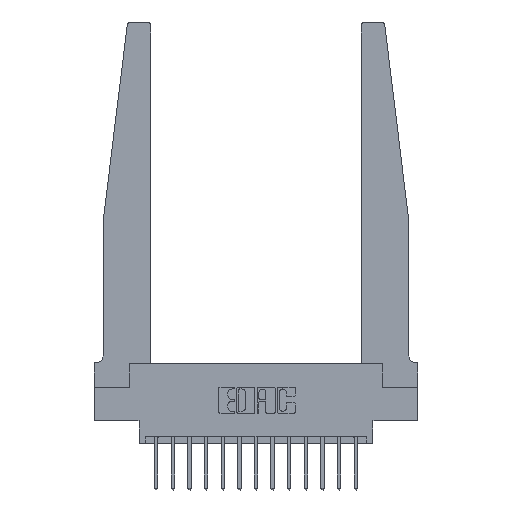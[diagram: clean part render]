
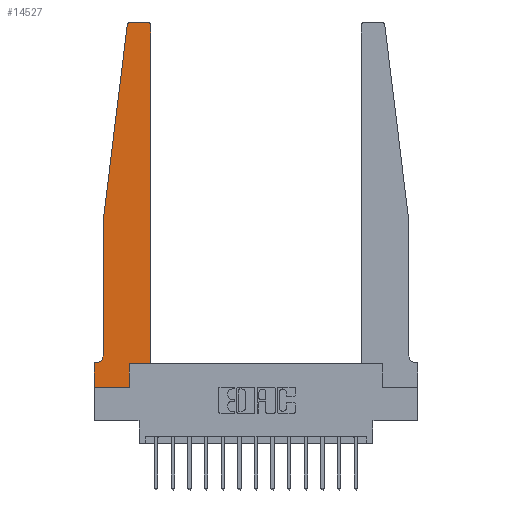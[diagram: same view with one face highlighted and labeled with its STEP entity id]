
A CAD part, top view. The second image highlights one B-rep face of the part: STEP entity #14527.
In plain terms, the highlighted planar face has unit normal (0, 0, 1).
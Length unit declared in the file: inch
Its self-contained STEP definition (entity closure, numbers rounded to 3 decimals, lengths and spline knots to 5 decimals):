
#249 = CARTESIAN_POINT ( 'NONE',  ( 0.2605, 0.18, 0.37 ) ) ;
#412 = VERTEX_POINT ( 'NONE', #7031 ) ;
#524 = DIRECTION ( 'NONE',  ( 1., 0., 0. ) ) ;
#553 = DIRECTION ( 'NONE',  ( -1., 0., 0. ) ) ;
#1362 = LINE ( 'NONE', #14492, #8134 ) ;
#2396 = CARTESIAN_POINT ( 'NONE',  ( 0.27653, 2.72, 0.37 ) ) ;
#2543 = DIRECTION ( 'NONE',  ( 1., 0., 0. ) ) ;
#2565 = VERTEX_POINT ( 'NONE', #249 ) ;
#2667 = EDGE_LOOP ( 'NONE', ( #16697, #17118, #3313, #10289, #3746, #11726, #4587, #15680, #12146, #9450, #15894, #10908 ) ) ;
#2703 = DIRECTION ( 'NONE',  ( 0., 0., -1. ) ) ;
#2817 = VECTOR ( 'NONE', #12743, 39.37008 ) ;
#2954 = AXIS2_PLACEMENT_3D ( 'NONE', #10752, #2703, #12099 ) ;
#3021 = EDGE_CURVE ( 'NONE', #12821, #3714, #10484, .T. ) ;
#3313 = ORIENTED_EDGE ( 'NONE', *, *, #9236, .T. ) ;
#3453 = VECTOR ( 'NONE', #9920, 39.37008 ) ;
#3548 = LINE ( 'NONE', #11405, #10287 ) ;
#3714 = VERTEX_POINT ( 'NONE', #16262 ) ;
#3727 = FACE_OUTER_BOUND ( 'NONE', #2667, .T. ) ;
#3746 = ORIENTED_EDGE ( 'NONE', *, *, #3021, .T. ) ;
#3760 = DIRECTION ( 'NONE',  ( 1., 0., 0. ) ) ;
#4009 = DIRECTION ( 'NONE',  ( 0., -1., 0. ) ) ;
#4229 = VERTEX_POINT ( 'NONE', #16012 ) ;
#4432 = VERTEX_POINT ( 'NONE', #14470 ) ;
#4587 = ORIENTED_EDGE ( 'NONE', *, *, #8149, .T. ) ;
#4724 = CARTESIAN_POINT ( 'NONE',  ( 0.2605, 0.18, 0.37 ) ) ;
#4730 = LINE ( 'NONE', #10599, #11858 ) ;
#5122 = EDGE_CURVE ( 'NONE', #2565, #16673, #4730, .T. ) ;
#5368 = VERTEX_POINT ( 'NONE', #8554 ) ;
#5575 = EDGE_CURVE ( 'NONE', #4432, #5368, #1362, .T. ) ;
#5915 = LINE ( 'NONE', #12047, #12614 ) ;
#6221 = VERTEX_POINT ( 'NONE', #14526 ) ;
#6348 = VECTOR ( 'NONE', #15197, 39.37008 ) ;
#6375 = CIRCLE ( 'NONE', #12359, 0.03 ) ;
#6402 = VERTEX_POINT ( 'NONE', #6806 ) ;
#6451 = EDGE_CURVE ( 'NONE', #16673, #6221, #14570, .T. ) ;
#6667 = AXIS2_PLACEMENT_3D ( 'NONE', #7241, #8604, #524 ) ;
#6700 = DIRECTION ( 'NONE',  ( 0., 0., 1. ) ) ;
#6715 = EDGE_CURVE ( 'NONE', #5368, #2565, #6821, .T. ) ;
#6806 = CARTESIAN_POINT ( 'NONE',  ( 0., 0.1875, 0.37 ) ) ;
#6821 = LINE ( 'NONE', #4724, #2817 ) ;
#6932 = AXIS2_PLACEMENT_3D ( 'NONE', #2396, #11792, #3760 ) ;
#7011 = CARTESIAN_POINT ( 'NONE',  ( 0.065, 0.2375, 0.37 ) ) ;
#7031 = CARTESIAN_POINT ( 'NONE',  ( 0.24675, 2.72367, 0.37 ) ) ;
#7032 = LINE ( 'NONE', #15213, #3453 ) ;
#7241 = CARTESIAN_POINT ( 'NONE',  ( 0., 0.1875, 0.37 ) ) ;
#7588 = EDGE_CURVE ( 'NONE', #12906, #11957, #15149, .T. ) ;
#7838 = DIRECTION ( 'NONE',  ( 1., 0., 0. ) ) ;
#8134 = VECTOR ( 'NONE', #7838, 39.37008 ) ;
#8149 = EDGE_CURVE ( 'NONE', #6402, #4432, #10353, .T. ) ;
#8226 = CARTESIAN_POINT ( 'NONE',  ( 0.425, 0.18, 0.37 ) ) ;
#8378 = CIRCLE ( 'NONE', #6932, 0.03 ) ;
#8470 = CARTESIAN_POINT ( 'NONE',  ( 0.27653, 2.75, 0.37 ) ) ;
#8554 = CARTESIAN_POINT ( 'NONE',  ( 0.2605, 0., 0.37 ) ) ;
#8604 = DIRECTION ( 'NONE',  ( 0., 0., 1. ) ) ;
#9236 = EDGE_CURVE ( 'NONE', #412, #4229, #7032, .T. ) ;
#9450 = ORIENTED_EDGE ( 'NONE', *, *, #5122, .T. ) ;
#9846 = CARTESIAN_POINT ( 'NONE',  ( 0., 0., 0.37 ) ) ;
#9920 = DIRECTION ( 'NONE',  ( -0.122, -0.992, 0. ) ) ;
#10068 = EDGE_CURVE ( 'NONE', #6221, #12906, #6375, .T. ) ;
#10287 = VECTOR ( 'NONE', #12667, 39.37008 ) ;
#10289 = ORIENTED_EDGE ( 'NONE', *, *, #11103, .T. ) ;
#10353 = LINE ( 'NONE', #9846, #6348 ) ;
#10484 = CIRCLE ( 'NONE', #2954, 0.05 ) ;
#10599 = CARTESIAN_POINT ( 'NONE',  ( 0.425, 0.18, 0.37 ) ) ;
#10752 = CARTESIAN_POINT ( 'NONE',  ( 0.015, 0.2375, 0.37 ) ) ;
#10902 = DIRECTION ( 'NONE',  ( 0., 1., 0. ) ) ;
#10908 = ORIENTED_EDGE ( 'NONE', *, *, #10068, .T. ) ;
#11103 = EDGE_CURVE ( 'NONE', #4229, #12821, #5915, .T. ) ;
#11405 = CARTESIAN_POINT ( 'NONE',  ( 0.065, 0.1875, 0.37 ) ) ;
#11726 = ORIENTED_EDGE ( 'NONE', *, *, #12977, .T. ) ;
#11792 = DIRECTION ( 'NONE',  ( 0., 0., 1. ) ) ;
#11804 = CARTESIAN_POINT ( 'NONE',  ( 0.425, 0.18, 0.37 ) ) ;
#11858 = VECTOR ( 'NONE', #2543, 39.37008 ) ;
#11957 = VERTEX_POINT ( 'NONE', #8470 ) ;
#12047 = CARTESIAN_POINT ( 'NONE',  ( 0.065, 1.25, 0.37 ) ) ;
#12099 = DIRECTION ( 'NONE',  ( -1., 0., 0. ) ) ;
#12146 = ORIENTED_EDGE ( 'NONE', *, *, #6715, .T. ) ;
#12359 = AXIS2_PLACEMENT_3D ( 'NONE', #14709, #6700, #16029 ) ;
#12614 = VECTOR ( 'NONE', #4009, 39.37008 ) ;
#12667 = DIRECTION ( 'NONE',  ( -1., 0., 0. ) ) ;
#12743 = DIRECTION ( 'NONE',  ( 0., 1., 0. ) ) ;
#12821 = VERTEX_POINT ( 'NONE', #7011 ) ;
#12906 = VERTEX_POINT ( 'NONE', #16514 ) ;
#12977 = EDGE_CURVE ( 'NONE', #3714, #6402, #3548, .T. ) ;
#13300 = VECTOR ( 'NONE', #10902, 39.37008 ) ;
#14331 = VECTOR ( 'NONE', #553, 39.37008 ) ;
#14470 = CARTESIAN_POINT ( 'NONE',  ( 0., 0., 0.37 ) ) ;
#14492 = CARTESIAN_POINT ( 'NONE',  ( 0., 0., 0.37 ) ) ;
#14526 = CARTESIAN_POINT ( 'NONE',  ( 0.425, 2.72, 0.37 ) ) ;
#14527 = ADVANCED_FACE ( 'NONE', ( #3727 ), #15239, .T. ) ;
#14570 = LINE ( 'NONE', #8226, #13300 ) ;
#14709 = CARTESIAN_POINT ( 'NONE',  ( 0.395, 2.72, 0.37 ) ) ;
#15149 = LINE ( 'NONE', #15276, #14331 ) ;
#15197 = DIRECTION ( 'NONE',  ( 0., -1., 0. ) ) ;
#15213 = CARTESIAN_POINT ( 'NONE',  ( 0.065, 1.25, 0.37 ) ) ;
#15239 = PLANE ( 'NONE',  #6667 ) ;
#15276 = CARTESIAN_POINT ( 'NONE',  ( 0.25, 2.75, 0.37 ) ) ;
#15680 = ORIENTED_EDGE ( 'NONE', *, *, #5575, .T. ) ;
#15894 = ORIENTED_EDGE ( 'NONE', *, *, #6451, .T. ) ;
#16012 = CARTESIAN_POINT ( 'NONE',  ( 0.065, 1.25, 0.37 ) ) ;
#16029 = DIRECTION ( 'NONE',  ( 1., 0., 0. ) ) ;
#16262 = CARTESIAN_POINT ( 'NONE',  ( 0.015, 0.1875, 0.37 ) ) ;
#16514 = CARTESIAN_POINT ( 'NONE',  ( 0.395, 2.75, 0.37 ) ) ;
#16673 = VERTEX_POINT ( 'NONE', #11804 ) ;
#16697 = ORIENTED_EDGE ( 'NONE', *, *, #7588, .T. ) ;
#17118 = ORIENTED_EDGE ( 'NONE', *, *, #17240, .T. ) ;
#17240 = EDGE_CURVE ( 'NONE', #11957, #412, #8378, .T. ) ;
